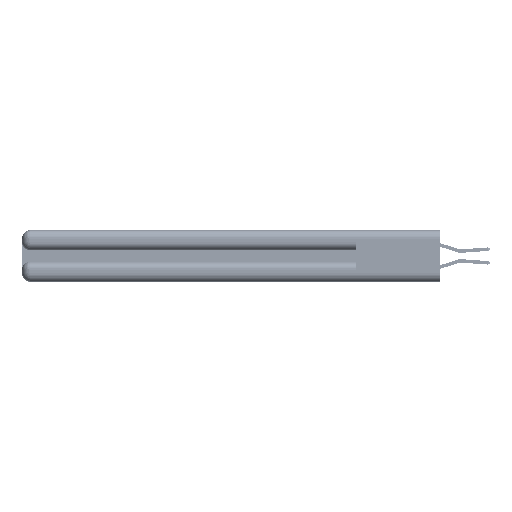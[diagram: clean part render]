
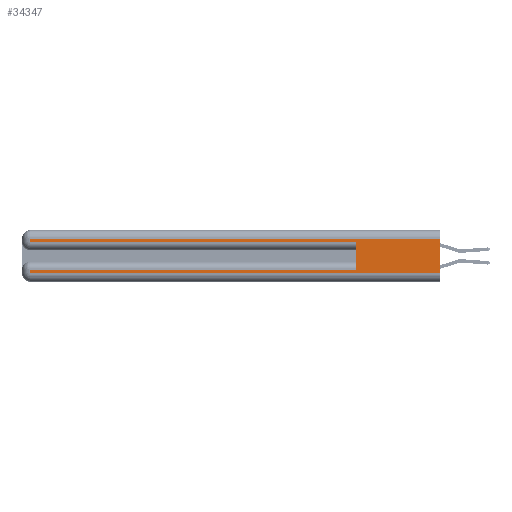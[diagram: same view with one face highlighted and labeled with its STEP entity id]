
A CAD part, left-side view. The second image highlights one B-rep face of the part: STEP entity #34347.
In plain terms, the highlighted planar face has unit normal (-1, 0, 0).
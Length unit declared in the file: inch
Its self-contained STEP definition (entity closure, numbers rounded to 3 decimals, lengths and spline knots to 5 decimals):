
#1091 = VECTOR ( 'NONE', #44984, 39.37008 ) ;
#1224 = ORIENTED_EDGE ( 'NONE', *, *, #36173, .T. ) ;
#1845 = CARTESIAN_POINT ( 'NONE',  ( 0., 0., 0.06 ) ) ;
#2037 = AXIS2_PLACEMENT_3D ( 'NONE', #25923, #30136, #4285 ) ;
#2223 = DIRECTION ( 'NONE',  ( 0., 1., 0. ) ) ;
#2356 = VERTEX_POINT ( 'NONE', #46595 ) ;
#3068 = CARTESIAN_POINT ( 'NONE',  ( 0., 0.6, 0.145 ) ) ;
#3195 = CARTESIAN_POINT ( 'NONE',  ( 0., 0., 0.31 ) ) ;
#3317 = EDGE_CURVE ( 'NONE', #37730, #10396, #17567, .T. ) ;
#3955 = LINE ( 'NONE', #18359, #48450 ) ;
#4285 = DIRECTION ( 'NONE',  ( 0., 0., -1. ) ) ;
#5238 = CARTESIAN_POINT ( 'NONE',  ( 0., 0., 0.37 ) ) ;
#6305 = VECTOR ( 'NONE', #2223, 39.37008 ) ;
#7368 = DIRECTION ( 'NONE',  ( 0., 0., 1. ) ) ;
#9350 = CARTESIAN_POINT ( 'NONE',  ( 0., 2.94, 0.37 ) ) ;
#9714 = ORIENTED_EDGE ( 'NONE', *, *, #26009, .T. ) ;
#10396 = VERTEX_POINT ( 'NONE', #26597 ) ;
#12231 = CARTESIAN_POINT ( 'NONE',  ( 0., 2.94, 0.06 ) ) ;
#13189 = EDGE_CURVE ( 'NONE', #27535, #10396, #38217, .T. ) ;
#13498 = CARTESIAN_POINT ( 'NONE',  ( 0., 0., 0.285 ) ) ;
#14400 = EDGE_CURVE ( 'NONE', #2356, #27535, #3955, .T. ) ;
#15064 = ORIENTED_EDGE ( 'NONE', *, *, #3317, .F. ) ;
#15144 = CARTESIAN_POINT ( 'NONE',  ( 0., 2.94, 0.31 ) ) ;
#15209 = CARTESIAN_POINT ( 'NONE',  ( 0., 0., 0.085 ) ) ;
#16429 = VERTEX_POINT ( 'NONE', #15144 ) ;
#17567 = LINE ( 'NONE', #5238, #26354 ) ;
#17768 = CARTESIAN_POINT ( 'NONE',  ( 0., 0.6, 0.085 ) ) ;
#17854 = DIRECTION ( 'NONE',  ( 0., -1., 0. ) ) ;
#18359 = CARTESIAN_POINT ( 'NONE',  ( 0., 2.94, 0.37 ) ) ;
#22021 = EDGE_CURVE ( 'NONE', #25062, #26269, #22955, .T. ) ;
#22642 = ORIENTED_EDGE ( 'NONE', *, *, #48782, .T. ) ;
#22781 = ORIENTED_EDGE ( 'NONE', *, *, #36473, .T. ) ;
#22955 = LINE ( 'NONE', #3068, #44515 ) ;
#25062 = VERTEX_POINT ( 'NONE', #17768 ) ;
#25923 = CARTESIAN_POINT ( 'NONE',  ( 0., 0., 0.37 ) ) ;
#26009 = EDGE_CURVE ( 'NONE', #25062, #2356, #50817, .T. ) ;
#26269 = VERTEX_POINT ( 'NONE', #34433 ) ;
#26354 = VECTOR ( 'NONE', #44034, 39.37008 ) ;
#26597 = CARTESIAN_POINT ( 'NONE',  ( 0., 0., 0.06 ) ) ;
#27485 = EDGE_LOOP ( 'NONE', ( #15064, #1224, #22642, #22781, #39409, #9714, #29241, #32710 ) ) ;
#27535 = VERTEX_POINT ( 'NONE', #12231 ) ;
#29241 = ORIENTED_EDGE ( 'NONE', *, *, #14400, .T. ) ;
#30136 = DIRECTION ( 'NONE',  ( 1., 0., 0. ) ) ;
#30601 = CARTESIAN_POINT ( 'NONE',  ( 0., 0., 0.31 ) ) ;
#31351 = LINE ( 'NONE', #3195, #52866 ) ;
#32710 = ORIENTED_EDGE ( 'NONE', *, *, #13189, .T. ) ;
#33359 = DIRECTION ( 'NONE',  ( 0., 1., 0. ) ) ;
#34347 = ADVANCED_FACE ( 'NONE', ( #50989 ), #47245, .F. ) ;
#34433 = CARTESIAN_POINT ( 'NONE',  ( 0., 0.6, 0.285 ) ) ;
#35383 = DIRECTION ( 'NONE',  ( 0., 0., -1. ) ) ;
#36173 = EDGE_CURVE ( 'NONE', #37730, #16429, #31351, .T. ) ;
#36473 = EDGE_CURVE ( 'NONE', #50144, #26269, #49458, .T. ) ;
#36677 = VECTOR ( 'NONE', #17854, 39.37008 ) ;
#37730 = VERTEX_POINT ( 'NONE', #30601 ) ;
#38217 = LINE ( 'NONE', #1845, #1091 ) ;
#39409 = ORIENTED_EDGE ( 'NONE', *, *, #22021, .F. ) ;
#40043 = DIRECTION ( 'NONE',  ( 0., 0., -1. ) ) ;
#40336 = CARTESIAN_POINT ( 'NONE',  ( 0., 2.94, 0.285 ) ) ;
#43981 = VECTOR ( 'NONE', #35383, 39.37008 ) ;
#44034 = DIRECTION ( 'NONE',  ( 0., 0., -1. ) ) ;
#44515 = VECTOR ( 'NONE', #7368, 39.37008 ) ;
#44984 = DIRECTION ( 'NONE',  ( 0., -1., 0. ) ) ;
#46595 = CARTESIAN_POINT ( 'NONE',  ( 0., 2.94, 0.085 ) ) ;
#47245 = PLANE ( 'NONE',  #2037 ) ;
#48450 = VECTOR ( 'NONE', #40043, 39.37008 ) ;
#48782 = EDGE_CURVE ( 'NONE', #16429, #50144, #55438, .T. ) ;
#49458 = LINE ( 'NONE', #13498, #36677 ) ;
#50144 = VERTEX_POINT ( 'NONE', #40336 ) ;
#50817 = LINE ( 'NONE', #15209, #6305 ) ;
#50989 = FACE_OUTER_BOUND ( 'NONE', #27485, .T. ) ;
#52866 = VECTOR ( 'NONE', #33359, 39.37008 ) ;
#55438 = LINE ( 'NONE', #9350, #43981 ) ;
